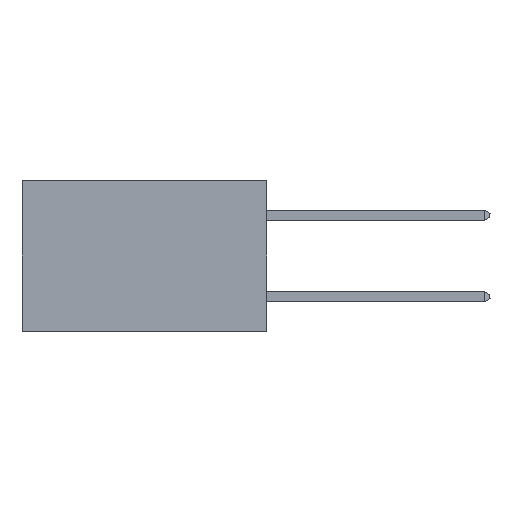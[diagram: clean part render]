
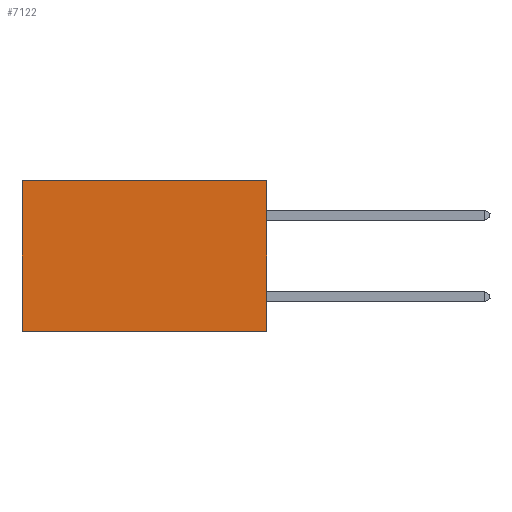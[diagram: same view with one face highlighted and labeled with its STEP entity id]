
A CAD part, left-side view. The second image highlights one B-rep face of the part: STEP entity #7122.
In plain terms, the highlighted planar face has unit normal (-1, 0, 0).
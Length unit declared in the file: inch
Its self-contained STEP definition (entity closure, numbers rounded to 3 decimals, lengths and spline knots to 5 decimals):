
#458 = CARTESIAN_POINT ( 'NONE',  ( 0.2875, 0.6, 0. ) ) ;
#3540 = LINE ( 'NONE', #34434, #18157 ) ;
#3951 = VERTEX_POINT ( 'NONE', #458 ) ;
#4722 = ORIENTED_EDGE ( 'NONE', *, *, #18346, .T. ) ;
#6127 = CARTESIAN_POINT ( 'NONE',  ( 0.2875, 0., -0.37 ) ) ;
#6239 = PLANE ( 'NONE',  #15176 ) ;
#7122 = ADVANCED_FACE ( 'NONE', ( #9983 ), #6239, .F. ) ;
#7395 = DIRECTION ( 'NONE',  ( 0., 1., 0. ) ) ;
#7542 = CARTESIAN_POINT ( 'NONE',  ( 0.2875, 0., 0. ) ) ;
#9179 = DIRECTION ( 'NONE',  ( 1., 0., 0. ) ) ;
#9299 = EDGE_CURVE ( 'NONE', #21627, #37246, #30626, .T. ) ;
#9983 = FACE_OUTER_BOUND ( 'NONE', #11516, .T. ) ;
#10471 = CARTESIAN_POINT ( 'NONE',  ( 0.2875, 0., 0. ) ) ;
#11516 = EDGE_LOOP ( 'NONE', ( #26367, #31740, #31559, #4722 ) ) ;
#12333 = VECTOR ( 'NONE', #7395, 39.37008 ) ;
#15176 = AXIS2_PLACEMENT_3D ( 'NONE', #32930, #9179, #29536 ) ;
#16861 = DIRECTION ( 'NONE',  ( 0., 0., -1. ) ) ;
#18157 = VECTOR ( 'NONE', #21881, 39.37008 ) ;
#18346 = EDGE_CURVE ( 'NONE', #38986, #3951, #31079, .T. ) ;
#19734 = CARTESIAN_POINT ( 'NONE',  ( 0.2875, 0., 0. ) ) ;
#21627 = VERTEX_POINT ( 'NONE', #23334 ) ;
#21881 = DIRECTION ( 'NONE',  ( 0., 0., -1. ) ) ;
#23334 = CARTESIAN_POINT ( 'NONE',  ( 0.2875, 0., -0.37 ) ) ;
#26367 = ORIENTED_EDGE ( 'NONE', *, *, #42845, .T. ) ;
#29130 = DIRECTION ( 'NONE',  ( 0., 1., 0. ) ) ;
#29536 = DIRECTION ( 'NONE',  ( 0., 0., -1. ) ) ;
#30626 = LINE ( 'NONE', #6127, #38435 ) ;
#31079 = LINE ( 'NONE', #7542, #12333 ) ;
#31099 = CARTESIAN_POINT ( 'NONE',  ( 0.2875, 0.6, -0.37 ) ) ;
#31559 = ORIENTED_EDGE ( 'NONE', *, *, #32405, .F. ) ;
#31740 = ORIENTED_EDGE ( 'NONE', *, *, #9299, .F. ) ;
#32405 = EDGE_CURVE ( 'NONE', #38986, #21627, #37273, .T. ) ;
#32930 = CARTESIAN_POINT ( 'NONE',  ( 0.2875, 0., 0. ) ) ;
#34434 = CARTESIAN_POINT ( 'NONE',  ( 0.2875, 0.6, 0. ) ) ;
#36705 = VECTOR ( 'NONE', #16861, 39.37008 ) ;
#37246 = VERTEX_POINT ( 'NONE', #31099 ) ;
#37273 = LINE ( 'NONE', #10471, #36705 ) ;
#38435 = VECTOR ( 'NONE', #29130, 39.37008 ) ;
#38986 = VERTEX_POINT ( 'NONE', #19734 ) ;
#42845 = EDGE_CURVE ( 'NONE', #3951, #37246, #3540, .T. ) ;
